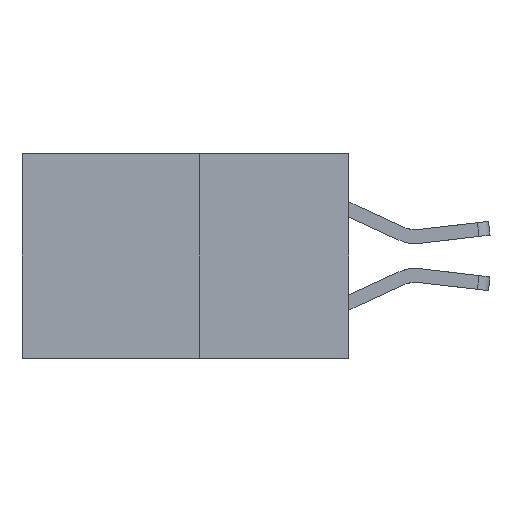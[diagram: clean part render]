
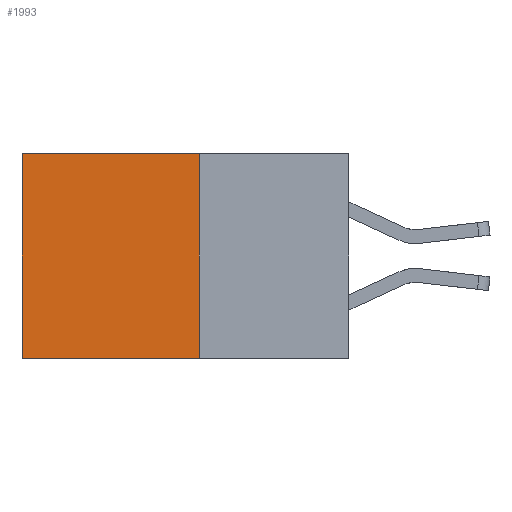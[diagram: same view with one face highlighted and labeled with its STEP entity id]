
A CAD part, left-side view. The second image highlights one B-rep face of the part: STEP entity #1993.
In plain terms, the highlighted planar face has unit normal (-1, 0, 0).
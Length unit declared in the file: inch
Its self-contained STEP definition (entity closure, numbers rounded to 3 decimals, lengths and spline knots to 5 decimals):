
#23 = CARTESIAN_POINT ( 'NONE',  ( 0.277, 0.59, -0.37 ) ) ;
#534 = DIRECTION ( 'NONE',  ( 0., 0., -1. ) ) ;
#570 = LINE ( 'NONE', #3437, #2821 ) ;
#573 = CARTESIAN_POINT ( 'NONE',  ( 0.277, 0.59, -0.37 ) ) ;
#1806 = VERTEX_POINT ( 'NONE', #10152 ) ;
#1993 = ADVANCED_FACE ( 'NONE', ( #3964 ), #2559, .F. ) ;
#2517 = DIRECTION ( 'NONE',  ( 0., 1., 0. ) ) ;
#2559 = PLANE ( 'NONE',  #3005 ) ;
#2627 = CARTESIAN_POINT ( 'NONE',  ( 0.277, 0.27, -0.37 ) ) ;
#2821 = VECTOR ( 'NONE', #6952, 39.37008 ) ;
#3005 = AXIS2_PLACEMENT_3D ( 'NONE', #11005, #5474, #3972 ) ;
#3285 = EDGE_CURVE ( 'NONE', #1806, #3541, #5264, .T. ) ;
#3437 = CARTESIAN_POINT ( 'NONE',  ( 0.277, 0.27, -0.37 ) ) ;
#3541 = VERTEX_POINT ( 'NONE', #6273 ) ;
#3964 = FACE_OUTER_BOUND ( 'NONE', #6049, .T. ) ;
#3972 = DIRECTION ( 'NONE',  ( 0., 0., -1. ) ) ;
#4244 = ORIENTED_EDGE ( 'NONE', *, *, #3285, .T. ) ;
#4792 = EDGE_CURVE ( 'NONE', #10573, #7281, #9673, .T. ) ;
#5264 = LINE ( 'NONE', #10031, #5548 ) ;
#5474 = DIRECTION ( 'NONE',  ( 1., 0., 0. ) ) ;
#5548 = VECTOR ( 'NONE', #9722, 39.37008 ) ;
#6049 = EDGE_LOOP ( 'NONE', ( #8914, #6607, #6392, #4244 ) ) ;
#6273 = CARTESIAN_POINT ( 'NONE',  ( 0.277, 0.59, 0. ) ) ;
#6392 = ORIENTED_EDGE ( 'NONE', *, *, #9315, .F. ) ;
#6607 = ORIENTED_EDGE ( 'NONE', *, *, #4792, .F. ) ;
#6905 = VECTOR ( 'NONE', #534, 39.37008 ) ;
#6952 = DIRECTION ( 'NONE',  ( 0., 0., -1. ) ) ;
#7224 = EDGE_CURVE ( 'NONE', #3541, #7281, #11246, .T. ) ;
#7281 = VERTEX_POINT ( 'NONE', #23 ) ;
#7362 = CARTESIAN_POINT ( 'NONE',  ( 0.277, 0.27, -0.37 ) ) ;
#7458 = VECTOR ( 'NONE', #2517, 39.37008 ) ;
#8914 = ORIENTED_EDGE ( 'NONE', *, *, #7224, .T. ) ;
#9315 = EDGE_CURVE ( 'NONE', #1806, #10573, #570, .T. ) ;
#9673 = LINE ( 'NONE', #2627, #7458 ) ;
#9722 = DIRECTION ( 'NONE',  ( 0., 1., 0. ) ) ;
#10031 = CARTESIAN_POINT ( 'NONE',  ( 0.277, 0.27, 0. ) ) ;
#10152 = CARTESIAN_POINT ( 'NONE',  ( 0.277, 0.27, 0. ) ) ;
#10573 = VERTEX_POINT ( 'NONE', #7362 ) ;
#11005 = CARTESIAN_POINT ( 'NONE',  ( 0.277, 0.27, -0.37 ) ) ;
#11246 = LINE ( 'NONE', #573, #6905 ) ;
